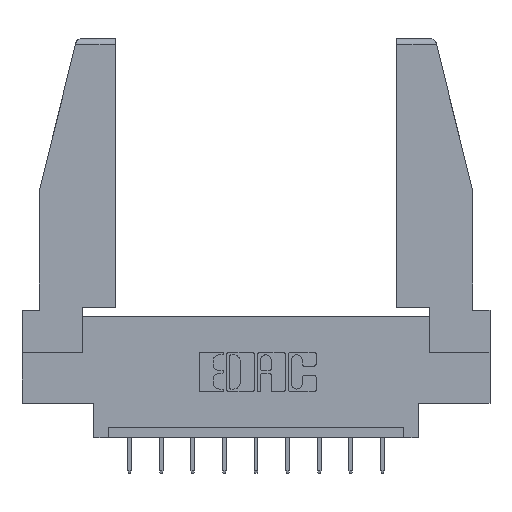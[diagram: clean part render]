
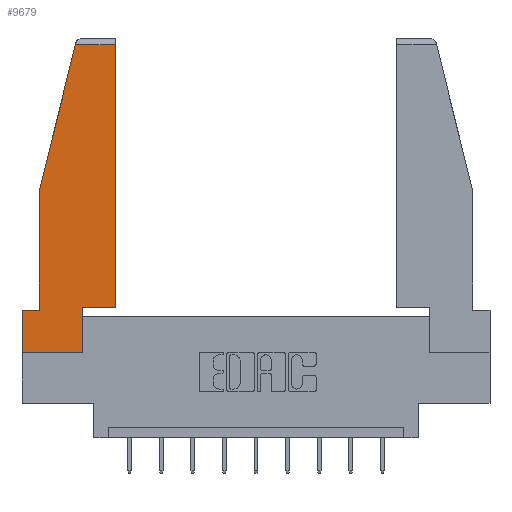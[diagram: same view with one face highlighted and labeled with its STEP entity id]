
A CAD part, top view. The second image highlights one B-rep face of the part: STEP entity #9679.
In plain terms, the highlighted planar face has unit normal (0, 0, 1).
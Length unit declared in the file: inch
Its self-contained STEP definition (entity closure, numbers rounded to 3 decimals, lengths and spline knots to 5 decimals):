
#77 = VECTOR ( 'NONE', #8485, 39.37008 ) ;
#246 = DIRECTION ( 'NONE',  ( 0., -1., 0. ) ) ;
#283 = EDGE_CURVE ( 'NONE', #679, #6127, #13285, .T. ) ;
#444 = VECTOR ( 'NONE', #10949, 39.37008 ) ;
#652 = VERTEX_POINT ( 'NONE', #6066 ) ;
#679 = VERTEX_POINT ( 'NONE', #11842 ) ;
#710 = EDGE_CURVE ( 'NONE', #10654, #3790, #8996, .T. ) ;
#933 = VECTOR ( 'NONE', #246, 39.37008 ) ;
#1001 = VECTOR ( 'NONE', #1084, 39.37008 ) ;
#1084 = DIRECTION ( 'NONE',  ( -1., 0., 0. ) ) ;
#1264 = VECTOR ( 'NONE', #10269, 39.37008 ) ;
#1782 = CARTESIAN_POINT ( 'NONE',  ( 0.297, 0.223, 0. ) ) ;
#2222 = VERTEX_POINT ( 'NONE', #12835 ) ;
#2757 = ORIENTED_EDGE ( 'NONE', *, *, #12371, .T. ) ;
#3046 = EDGE_CURVE ( 'NONE', #8911, #652, #13329, .T. ) ;
#3088 = DIRECTION ( 'NONE',  ( -0.239, -0.971, 0. ) ) ;
#3115 = CARTESIAN_POINT ( 'NONE',  ( 0.297, 0., 0. ) ) ;
#3422 = CARTESIAN_POINT ( 'NONE',  ( 0.461, 0.223, 0. ) ) ;
#3790 = VERTEX_POINT ( 'NONE', #5177 ) ;
#3994 = CARTESIAN_POINT ( 'NONE',  ( 0.297, 0.223, 0. ) ) ;
#5177 = CARTESIAN_POINT ( 'NONE',  ( 0.086, 0.21, 0. ) ) ;
#5246 = CARTESIAN_POINT ( 'NONE',  ( 0., 1.52, 0. ) ) ;
#5537 = CARTESIAN_POINT ( 'NONE',  ( 0., 0.21, 0. ) ) ;
#5681 = CARTESIAN_POINT ( 'NONE',  ( 0., 0., 0. ) ) ;
#5811 = CARTESIAN_POINT ( 'NONE',  ( 0., 0.21, 0. ) ) ;
#5867 = ORIENTED_EDGE ( 'NONE', *, *, #9702, .T. ) ;
#5919 = DIRECTION ( 'NONE',  ( -1., 0., 0. ) ) ;
#5965 = VECTOR ( 'NONE', #6844, 39.37008 ) ;
#6066 = CARTESIAN_POINT ( 'NONE',  ( 0.461, 1.52, 0. ) ) ;
#6127 = VERTEX_POINT ( 'NONE', #10925 ) ;
#6298 = EDGE_CURVE ( 'NONE', #6127, #8757, #8618, .T. ) ;
#6306 = CARTESIAN_POINT ( 'NONE',  ( 0.271, 1.55, 0. ) ) ;
#6549 = ORIENTED_EDGE ( 'NONE', *, *, #710, .T. ) ;
#6844 = DIRECTION ( 'NONE',  ( 0., -1., 0. ) ) ;
#7064 = CARTESIAN_POINT ( 'NONE',  ( 0., 0.21, 0. ) ) ;
#7251 = ORIENTED_EDGE ( 'NONE', *, *, #10996, .T. ) ;
#7604 = LINE ( 'NONE', #5246, #1001 ) ;
#7768 = ORIENTED_EDGE ( 'NONE', *, *, #6298, .T. ) ;
#8041 = EDGE_LOOP ( 'NONE', ( #9400, #8361, #7251, #6549, #9925, #2757, #11335, #7768, #5867 ) ) ;
#8111 = VERTEX_POINT ( 'NONE', #5811 ) ;
#8163 = DIRECTION ( 'NONE',  ( 1., 0., 0. ) ) ;
#8361 = ORIENTED_EDGE ( 'NONE', *, *, #12927, .T. ) ;
#8485 = DIRECTION ( 'NONE',  ( 0., 1., 0. ) ) ;
#8618 = LINE ( 'NONE', #3115, #77 ) ;
#8757 = VERTEX_POINT ( 'NONE', #3994 ) ;
#8911 = VERTEX_POINT ( 'NONE', #3422 ) ;
#8971 = VECTOR ( 'NONE', #5919, 39.37008 ) ;
#8996 = LINE ( 'NONE', #12933, #933 ) ;
#9183 = PLANE ( 'NONE',  #10291 ) ;
#9400 = ORIENTED_EDGE ( 'NONE', *, *, #3046, .T. ) ;
#9679 = ADVANCED_FACE ( 'NONE', ( #11631 ), #9183, .T. ) ;
#9702 = EDGE_CURVE ( 'NONE', #8757, #8911, #12292, .T. ) ;
#9925 = ORIENTED_EDGE ( 'NONE', *, *, #11080, .T. ) ;
#9977 = LINE ( 'NONE', #7064, #8971 ) ;
#10269 = DIRECTION ( 'NONE',  ( 1., 0., 0. ) ) ;
#10291 = AXIS2_PLACEMENT_3D ( 'NONE', #13454, #12362, #8163 ) ;
#10654 = VERTEX_POINT ( 'NONE', #13397 ) ;
#10858 = DIRECTION ( 'NONE',  ( 0., 1., 0. ) ) ;
#10925 = CARTESIAN_POINT ( 'NONE',  ( 0.297, 0., 0. ) ) ;
#10949 = DIRECTION ( 'NONE',  ( 1., 0., 0. ) ) ;
#10996 = EDGE_CURVE ( 'NONE', #2222, #10654, #11779, .T. ) ;
#11080 = EDGE_CURVE ( 'NONE', #3790, #8111, #9977, .T. ) ;
#11335 = ORIENTED_EDGE ( 'NONE', *, *, #283, .T. ) ;
#11452 = VECTOR ( 'NONE', #3088, 39.37008 ) ;
#11631 = FACE_OUTER_BOUND ( 'NONE', #8041, .T. ) ;
#11779 = LINE ( 'NONE', #6306, #11452 ) ;
#11842 = CARTESIAN_POINT ( 'NONE',  ( 0., 0., 0. ) ) ;
#12292 = LINE ( 'NONE', #1782, #1264 ) ;
#12362 = DIRECTION ( 'NONE',  ( 0., 0., 1. ) ) ;
#12371 = EDGE_CURVE ( 'NONE', #8111, #679, #12390, .T. ) ;
#12390 = LINE ( 'NONE', #5537, #5965 ) ;
#12660 = VECTOR ( 'NONE', #10858, 39.37008 ) ;
#12808 = CARTESIAN_POINT ( 'NONE',  ( 0.461, 0.223, 0. ) ) ;
#12835 = CARTESIAN_POINT ( 'NONE',  ( 0.2636, 1.52, 0. ) ) ;
#12927 = EDGE_CURVE ( 'NONE', #652, #2222, #7604, .T. ) ;
#12933 = CARTESIAN_POINT ( 'NONE',  ( 0.086, 0.8, 0. ) ) ;
#13285 = LINE ( 'NONE', #5681, #444 ) ;
#13329 = LINE ( 'NONE', #12808, #12660 ) ;
#13397 = CARTESIAN_POINT ( 'NONE',  ( 0.086, 0.8, 0. ) ) ;
#13454 = CARTESIAN_POINT ( 'NONE',  ( 0., 0., 0. ) ) ;
